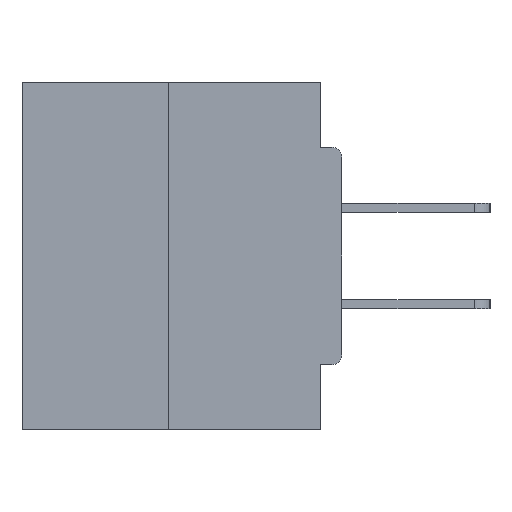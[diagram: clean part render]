
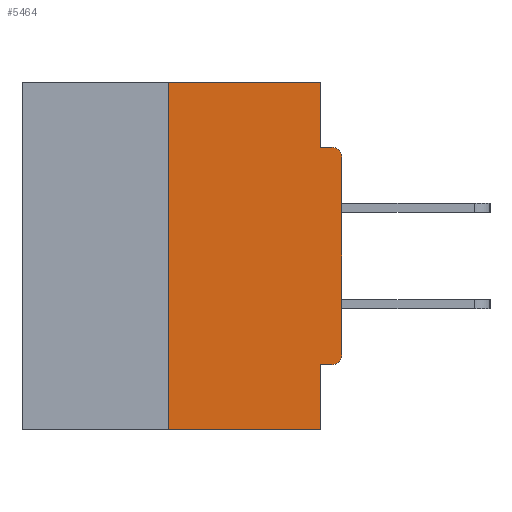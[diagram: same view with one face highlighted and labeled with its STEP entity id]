
A CAD part, left-side view. The second image highlights one B-rep face of the part: STEP entity #5464.
In plain terms, the highlighted planar face has unit normal (-1, 0, 0).
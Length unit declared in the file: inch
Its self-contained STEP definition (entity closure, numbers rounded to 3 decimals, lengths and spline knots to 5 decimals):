
#246 = EDGE_CURVE ( 'NONE', #1416, #7138, #20209, .T. ) ;
#1416 = VERTEX_POINT ( 'NONE', #10645 ) ;
#1695 = VERTEX_POINT ( 'NONE', #6900 ) ;
#2669 = EDGE_CURVE ( 'NONE', #30696, #1695, #19450, .T. ) ;
#2901 = AXIS2_PLACEMENT_3D ( 'NONE', #16898, #27357, #27908 ) ;
#2942 = EDGE_CURVE ( 'NONE', #4613, #4131, #30548, .T. ) ;
#3625 = ORIENTED_EDGE ( 'NONE', *, *, #5682, .F. ) ;
#3629 = ORIENTED_EDGE ( 'NONE', *, *, #17974, .F. ) ;
#4131 = VERTEX_POINT ( 'NONE', #29885 ) ;
#4154 = EDGE_CURVE ( 'NONE', #1695, #10793, #18977, .T. ) ;
#4326 = VECTOR ( 'NONE', #21162, 39.37008 ) ;
#4613 = VERTEX_POINT ( 'NONE', #26775 ) ;
#5116 = CARTESIAN_POINT ( 'NONE',  ( 0., 0.46, 0. ) ) ;
#5131 = CARTESIAN_POINT ( 'NONE',  ( 0., 0.25, 0. ) ) ;
#5279 = VECTOR ( 'NONE', #28032, 39.37008 ) ;
#5421 = CARTESIAN_POINT ( 'NONE',  ( 0., 0.031, -0.5 ) ) ;
#5464 = ADVANCED_FACE ( 'NONE', ( #7388 ), #12533, .F. ) ;
#5682 = EDGE_CURVE ( 'NONE', #25787, #11705, #6993, .T. ) ;
#5719 = VECTOR ( 'NONE', #30414, 39.37008 ) ;
#6496 = CARTESIAN_POINT ( 'NONE',  ( 0., 0.25, 0. ) ) ;
#6542 = AXIS2_PLACEMENT_3D ( 'NONE', #9774, #32377, #19722 ) ;
#6900 = CARTESIAN_POINT ( 'NONE',  ( 0., 0., -0.1085 ) ) ;
#6993 = LINE ( 'NONE', #5421, #14851 ) ;
#7043 = DIRECTION ( 'NONE',  ( 0., -1., 0. ) ) ;
#7138 = VERTEX_POINT ( 'NONE', #6496 ) ;
#7388 = FACE_OUTER_BOUND ( 'NONE', #25267, .T. ) ;
#7403 = DIRECTION ( 'NONE',  ( 0., 0., -1. ) ) ;
#7415 = CARTESIAN_POINT ( 'NONE',  ( 0., 0.46, -0.5 ) ) ;
#7512 = DIRECTION ( 'NONE',  ( -1., 0., 0. ) ) ;
#7876 = ORIENTED_EDGE ( 'NONE', *, *, #2942, .F. ) ;
#8589 = CARTESIAN_POINT ( 'NONE',  ( 0., 0.015, -0.0935 ) ) ;
#8622 = ORIENTED_EDGE ( 'NONE', *, *, #30062, .F. ) ;
#9684 = ORIENTED_EDGE ( 'NONE', *, *, #246, .F. ) ;
#9774 = CARTESIAN_POINT ( 'NONE',  ( 0., 0.46, 0. ) ) ;
#9887 = VECTOR ( 'NONE', #19040, 39.37008 ) ;
#10043 = CARTESIAN_POINT ( 'NONE',  ( 0., 0.031, -0.5 ) ) ;
#10559 = LINE ( 'NONE', #5116, #5719 ) ;
#10645 = CARTESIAN_POINT ( 'NONE',  ( 0., 0.25, -0.5 ) ) ;
#10793 = VERTEX_POINT ( 'NONE', #8589 ) ;
#11263 = LINE ( 'NONE', #7415, #5279 ) ;
#11409 = CARTESIAN_POINT ( 'NONE',  ( 0., 0., 0. ) ) ;
#11705 = VERTEX_POINT ( 'NONE', #10043 ) ;
#11712 = CARTESIAN_POINT ( 'NONE',  ( 0., 0., -0.0935 ) ) ;
#12533 = PLANE ( 'NONE',  #6542 ) ;
#12728 = VECTOR ( 'NONE', #14143, 39.37008 ) ;
#12841 = EDGE_CURVE ( 'NONE', #23719, #30696, #24962, .T. ) ;
#12949 = ORIENTED_EDGE ( 'NONE', *, *, #4154, .T. ) ;
#14143 = DIRECTION ( 'NONE',  ( 0., 0., 1. ) ) ;
#14851 = VECTOR ( 'NONE', #20259, 39.37008 ) ;
#15629 = EDGE_CURVE ( 'NONE', #1416, #11705, #11263, .T. ) ;
#16898 = CARTESIAN_POINT ( 'NONE',  ( 0., 0.015, -0.3915 ) ) ;
#17974 = EDGE_CURVE ( 'NONE', #23719, #25787, #19777, .T. ) ;
#18977 = CIRCLE ( 'NONE', #30749, 0.015 ) ;
#19040 = DIRECTION ( 'NONE',  ( 0., 1., 0. ) ) ;
#19387 = CARTESIAN_POINT ( 'NONE',  ( 0., 0.031, -0.4065 ) ) ;
#19450 = LINE ( 'NONE', #11409, #12728 ) ;
#19722 = DIRECTION ( 'NONE',  ( 0., 0., -1. ) ) ;
#19777 = LINE ( 'NONE', #26702, #9887 ) ;
#20209 = LINE ( 'NONE', #5131, #4326 ) ;
#20259 = DIRECTION ( 'NONE',  ( 0., 0., -1. ) ) ;
#20449 = ORIENTED_EDGE ( 'NONE', *, *, #2669, .T. ) ;
#21162 = DIRECTION ( 'NONE',  ( 0., 0., 1. ) ) ;
#21654 = ORIENTED_EDGE ( 'NONE', *, *, #15629, .T. ) ;
#23259 = CARTESIAN_POINT ( 'NONE',  ( 0., 0.015, -0.4065 ) ) ;
#23719 = VERTEX_POINT ( 'NONE', #23259 ) ;
#24391 = CARTESIAN_POINT ( 'NONE',  ( 0., 0., -0.3915 ) ) ;
#24555 = VECTOR ( 'NONE', #7403, 39.37008 ) ;
#24882 = VECTOR ( 'NONE', #7043, 39.37008 ) ;
#24962 = CIRCLE ( 'NONE', #2901, 0.015 ) ;
#25108 = CARTESIAN_POINT ( 'NONE',  ( 0., 0.031, 0. ) ) ;
#25267 = EDGE_LOOP ( 'NONE', ( #30230, #9684, #21654, #3625, #3629, #27427, #20449, #12949, #8622, #7876 ) ) ;
#25336 = CARTESIAN_POINT ( 'NONE',  ( 0., 0.015, -0.1085 ) ) ;
#25612 = EDGE_CURVE ( 'NONE', #7138, #4613, #10559, .T. ) ;
#25787 = VERTEX_POINT ( 'NONE', #19387 ) ;
#26702 = CARTESIAN_POINT ( 'NONE',  ( 0., 0., -0.4065 ) ) ;
#26775 = CARTESIAN_POINT ( 'NONE',  ( 0., 0.031, 0. ) ) ;
#27357 = DIRECTION ( 'NONE',  ( -1., 0., 0. ) ) ;
#27427 = ORIENTED_EDGE ( 'NONE', *, *, #12841, .T. ) ;
#27908 = DIRECTION ( 'NONE',  ( 0., 0., -1. ) ) ;
#28032 = DIRECTION ( 'NONE',  ( 0., -1., 0. ) ) ;
#29247 = LINE ( 'NONE', #11712, #24882 ) ;
#29885 = CARTESIAN_POINT ( 'NONE',  ( 0., 0.031, -0.0935 ) ) ;
#30062 = EDGE_CURVE ( 'NONE', #4131, #10793, #29247, .T. ) ;
#30230 = ORIENTED_EDGE ( 'NONE', *, *, #25612, .F. ) ;
#30414 = DIRECTION ( 'NONE',  ( 0., -1., 0. ) ) ;
#30548 = LINE ( 'NONE', #25108, #24555 ) ;
#30567 = DIRECTION ( 'NONE',  ( 0., 0., -1. ) ) ;
#30696 = VERTEX_POINT ( 'NONE', #24391 ) ;
#30749 = AXIS2_PLACEMENT_3D ( 'NONE', #25336, #7512, #30567 ) ;
#32377 = DIRECTION ( 'NONE',  ( 1., 0., 0. ) ) ;
